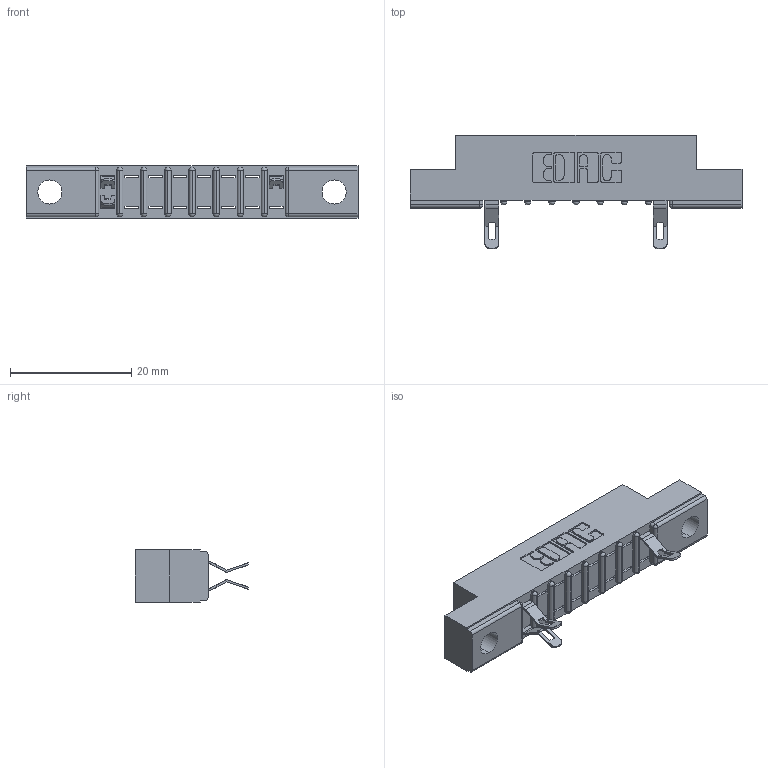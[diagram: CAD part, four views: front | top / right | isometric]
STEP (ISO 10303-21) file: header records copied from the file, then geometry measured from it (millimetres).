
FILE_DESCRIPTION (( 'STEP AP203' ), '1' );
FILE_NAME ('307-016-555-204.STEP', '2018-08-03T21:23:34', ( '' ), ( '' ), 'SwSTEP 2.0', 'SolidWorks 2016', '' );
FILE_SCHEMA (( 'CONFIG_CONTROL_DESIGN' ));
Length unit declared in the file: inch
Products named in the file (3): 307-290-001_555; 307-016-555-204; 307 Part_.156 Dia Mounting Holes
Assembly tree (4 placements, depth 2):
  307-016-555-204
    307 Part_.156 Dia Mounting Holes
    307-290-001_555  x3
Bounding box: 54.71 x 18.75 x 8.71 mm (x, y, z)
Volume: 3315 mm3; surface area: 4068.8 mm2
Topology: 4 solids, 4 shells, 454 faces, 1318 edges, 848 vertices
Faces by surface type: plane 264, cylinder 172, sphere 18
Entity records: 11845 total; most frequent: CARTESIAN_POINT 2013, ORIENTED_EDGE 2004, DIRECTION 1972, EDGE_CURVE 1002, VECTOR 750, LINE 750, VERTEX_POINT 652, AXIS2_PLACEMENT_3D 611
